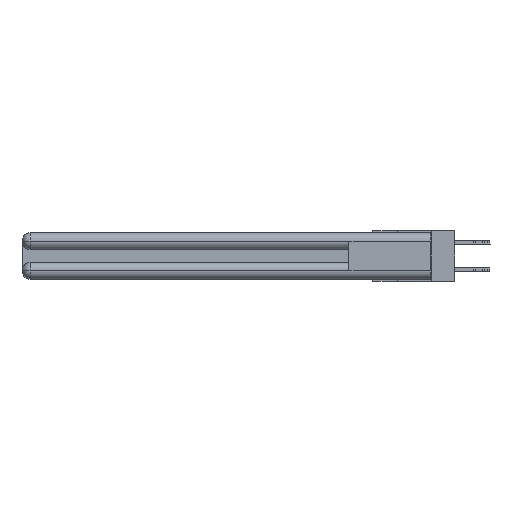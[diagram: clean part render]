
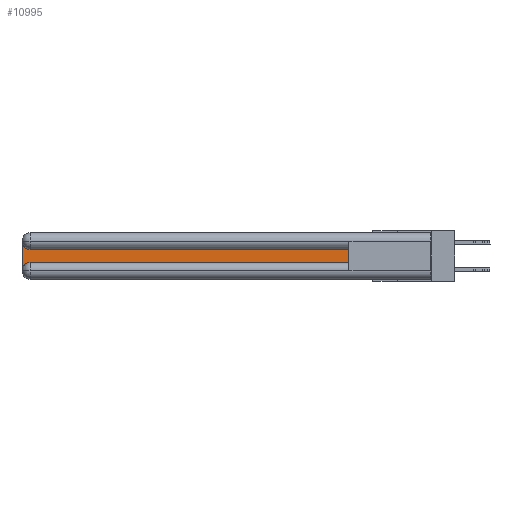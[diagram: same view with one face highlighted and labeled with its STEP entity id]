
A CAD part, left-side view. The second image highlights one B-rep face of the part: STEP entity #10995.
In plain terms, the highlighted planar face has unit normal (-1, 0, 0).
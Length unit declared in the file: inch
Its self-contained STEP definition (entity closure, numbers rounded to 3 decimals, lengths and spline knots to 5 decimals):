
#284 = LINE ( 'NONE', #20831, #17743 ) ;
#309 = DIRECTION ( 'NONE',  ( 1., 0., 0. ) ) ;
#1212 = CARTESIAN_POINT ( 'NONE',  ( 0.075, 2.94, -0.2175 ) ) ;
#1331 = CIRCLE ( 'NONE', #4887, 0.06 ) ;
#1782 = EDGE_LOOP ( 'NONE', ( #7359, #16178, #26435, #29539, #4079, #9353 ) ) ;
#2585 = EDGE_CURVE ( 'NONE', #6353, #13992, #31727, .T. ) ;
#4079 = ORIENTED_EDGE ( 'NONE', *, *, #7656, .T. ) ;
#4868 = VERTEX_POINT ( 'NONE', #17588 ) ;
#4887 = AXIS2_PLACEMENT_3D ( 'NONE', #17465, #309, #19948 ) ;
#4900 = CARTESIAN_POINT ( 'NONE',  ( 0.075, 3., -0.1225 ) ) ;
#6246 = CARTESIAN_POINT ( 'NONE',  ( 0.075, 0.6, -0.2175 ) ) ;
#6353 = VERTEX_POINT ( 'NONE', #15315 ) ;
#6781 = EDGE_CURVE ( 'NONE', #13992, #30112, #1331, .T. ) ;
#7359 = ORIENTED_EDGE ( 'NONE', *, *, #25343, .T. ) ;
#7656 = EDGE_CURVE ( 'NONE', #30112, #24035, #7832, .T. ) ;
#7832 = LINE ( 'NONE', #15334, #17548 ) ;
#9181 = FACE_OUTER_BOUND ( 'NONE', #1782, .T. ) ;
#9325 = CARTESIAN_POINT ( 'NONE',  ( 0.075, 3., -0.2775 ) ) ;
#9353 = ORIENTED_EDGE ( 'NONE', *, *, #24790, .T. ) ;
#9986 = DIRECTION ( 'NONE',  ( 0., 0., -1. ) ) ;
#10995 = ADVANCED_FACE ( 'NONE', ( #9181 ), #19745, .F. ) ;
#13093 = LINE ( 'NONE', #6246, #14687 ) ;
#13521 = CARTESIAN_POINT ( 'NONE',  ( 0.075, 2.94, -0.0625 ) ) ;
#13621 = DIRECTION ( 'NONE',  ( 0., 0., -1. ) ) ;
#13746 = DIRECTION ( 'NONE',  ( 0., 0., 1. ) ) ;
#13992 = VERTEX_POINT ( 'NONE', #9325 ) ;
#14687 = VECTOR ( 'NONE', #13746, 39.37008 ) ;
#15315 = CARTESIAN_POINT ( 'NONE',  ( 0.075, 3., -0.0625 ) ) ;
#15334 = CARTESIAN_POINT ( 'NONE',  ( 0.075, 0.6, -0.2175 ) ) ;
#16178 = ORIENTED_EDGE ( 'NONE', *, *, #31101, .T. ) ;
#16615 = DIRECTION ( 'NONE',  ( 0., 0., -1. ) ) ;
#16719 = CARTESIAN_POINT ( 'NONE',  ( 0.075, 3., -0.2175 ) ) ;
#17052 = DIRECTION ( 'NONE',  ( 1., 0., 0. ) ) ;
#17303 = VERTEX_POINT ( 'NONE', #21914 ) ;
#17465 = CARTESIAN_POINT ( 'NONE',  ( 0.075, 2.94, -0.2775 ) ) ;
#17548 = VECTOR ( 'NONE', #18455, 39.37008 ) ;
#17588 = CARTESIAN_POINT ( 'NONE',  ( 0.075, 2.94, -0.1225 ) ) ;
#17743 = VECTOR ( 'NONE', #30641, 39.37008 ) ;
#18455 = DIRECTION ( 'NONE',  ( 0., -1., 0. ) ) ;
#19745 = PLANE ( 'NONE',  #20537 ) ;
#19948 = DIRECTION ( 'NONE',  ( 0., 0., -1. ) ) ;
#20537 = AXIS2_PLACEMENT_3D ( 'NONE', #4900, #17052, #9986 ) ;
#20831 = CARTESIAN_POINT ( 'NONE',  ( 0.075, 0.6, -0.1225 ) ) ;
#21914 = CARTESIAN_POINT ( 'NONE',  ( 0.075, 0.6, -0.1225 ) ) ;
#23465 = DIRECTION ( 'NONE',  ( 1., 0., 0. ) ) ;
#24035 = VERTEX_POINT ( 'NONE', #30335 ) ;
#24790 = EDGE_CURVE ( 'NONE', #24035, #17303, #13093, .T. ) ;
#25343 = EDGE_CURVE ( 'NONE', #17303, #4868, #284, .T. ) ;
#25954 = VECTOR ( 'NONE', #16615, 39.37008 ) ;
#26435 = ORIENTED_EDGE ( 'NONE', *, *, #2585, .T. ) ;
#29539 = ORIENTED_EDGE ( 'NONE', *, *, #6781, .T. ) ;
#30112 = VERTEX_POINT ( 'NONE', #1212 ) ;
#30335 = CARTESIAN_POINT ( 'NONE',  ( 0.075, 0.6, -0.2175 ) ) ;
#30641 = DIRECTION ( 'NONE',  ( 0., 1., 0. ) ) ;
#31101 = EDGE_CURVE ( 'NONE', #4868, #6353, #31536, .T. ) ;
#31518 = AXIS2_PLACEMENT_3D ( 'NONE', #13521, #23465, #13621 ) ;
#31536 = CIRCLE ( 'NONE', #31518, 0.06 ) ;
#31727 = LINE ( 'NONE', #16719, #25954 ) ;
